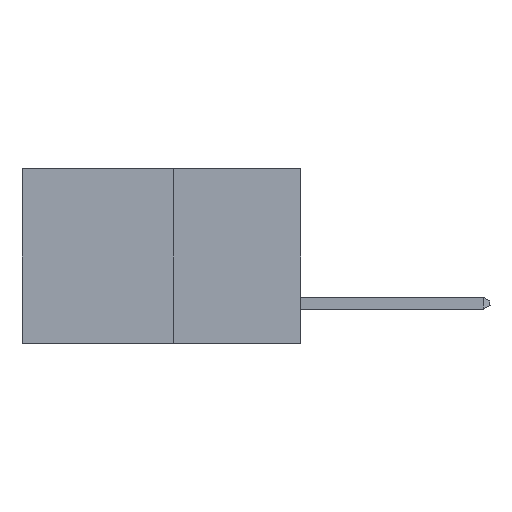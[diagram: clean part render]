
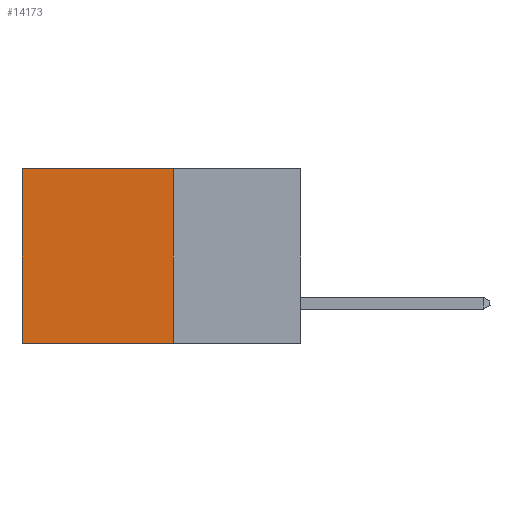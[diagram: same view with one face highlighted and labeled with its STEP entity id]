
A CAD part, left-side view. The second image highlights one B-rep face of the part: STEP entity #14173.
In plain terms, the highlighted planar face has unit normal (-1, 0, 0).
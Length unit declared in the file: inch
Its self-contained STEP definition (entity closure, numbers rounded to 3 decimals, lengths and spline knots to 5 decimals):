
#631 = DIRECTION ( 'NONE',  ( 1., 0., 0. ) ) ;
#1061 = VERTEX_POINT ( 'NONE', #15723 ) ;
#1339 = FACE_OUTER_BOUND ( 'NONE', #13642, .T. ) ;
#4273 = LINE ( 'NONE', #14320, #13250 ) ;
#4851 = DIRECTION ( 'NONE',  ( 0., 1., 0. ) ) ;
#5421 = AXIS2_PLACEMENT_3D ( 'NONE', #15617, #631, #12398 ) ;
#5537 = CARTESIAN_POINT ( 'NONE',  ( 0.277, 0.59, 0. ) ) ;
#5959 = DIRECTION ( 'NONE',  ( 0., 0., -1. ) ) ;
#6158 = VECTOR ( 'NONE', #14277, 39.37008 ) ;
#6265 = ORIENTED_EDGE ( 'NONE', *, *, #10704, .T. ) ;
#6545 = ORIENTED_EDGE ( 'NONE', *, *, #12968, .F. ) ;
#6976 = VERTEX_POINT ( 'NONE', #5537 ) ;
#8474 = EDGE_CURVE ( 'NONE', #20134, #16303, #19183, .T. ) ;
#8824 = VECTOR ( 'NONE', #10945, 39.37008 ) ;
#9954 = VECTOR ( 'NONE', #4851, 39.37008 ) ;
#10682 = LINE ( 'NONE', #12614, #6158 ) ;
#10704 = EDGE_CURVE ( 'NONE', #6976, #16303, #21346, .T. ) ;
#10739 = PLANE ( 'NONE',  #5421 ) ;
#10945 = DIRECTION ( 'NONE',  ( 0., 0., -1. ) ) ;
#11837 = ORIENTED_EDGE ( 'NONE', *, *, #12255, .T. ) ;
#12255 = EDGE_CURVE ( 'NONE', #1061, #6976, #10682, .T. ) ;
#12398 = DIRECTION ( 'NONE',  ( 0., 0., -1. ) ) ;
#12614 = CARTESIAN_POINT ( 'NONE',  ( 0.277, 0.27, 0. ) ) ;
#12968 = EDGE_CURVE ( 'NONE', #1061, #20134, #4273, .T. ) ;
#13250 = VECTOR ( 'NONE', #5959, 39.37008 ) ;
#13642 = EDGE_LOOP ( 'NONE', ( #6265, #15671, #6545, #11837 ) ) ;
#14168 = CARTESIAN_POINT ( 'NONE',  ( 0.277, 0.59, -0.37 ) ) ;
#14173 = ADVANCED_FACE ( 'NONE', ( #1339 ), #10739, .F. ) ;
#14277 = DIRECTION ( 'NONE',  ( 0., 1., 0. ) ) ;
#14320 = CARTESIAN_POINT ( 'NONE',  ( 0.277, 0.27, -0.37 ) ) ;
#14970 = CARTESIAN_POINT ( 'NONE',  ( 0.277, 0.27, -0.37 ) ) ;
#15617 = CARTESIAN_POINT ( 'NONE',  ( 0.277, 0.27, -0.37 ) ) ;
#15671 = ORIENTED_EDGE ( 'NONE', *, *, #8474, .F. ) ;
#15723 = CARTESIAN_POINT ( 'NONE',  ( 0.277, 0.27, 0. ) ) ;
#15836 = CARTESIAN_POINT ( 'NONE',  ( 0.277, 0.27, -0.37 ) ) ;
#16303 = VERTEX_POINT ( 'NONE', #14168 ) ;
#19183 = LINE ( 'NONE', #14970, #9954 ) ;
#20134 = VERTEX_POINT ( 'NONE', #15836 ) ;
#20698 = CARTESIAN_POINT ( 'NONE',  ( 0.277, 0.59, -0.37 ) ) ;
#21346 = LINE ( 'NONE', #20698, #8824 ) ;
